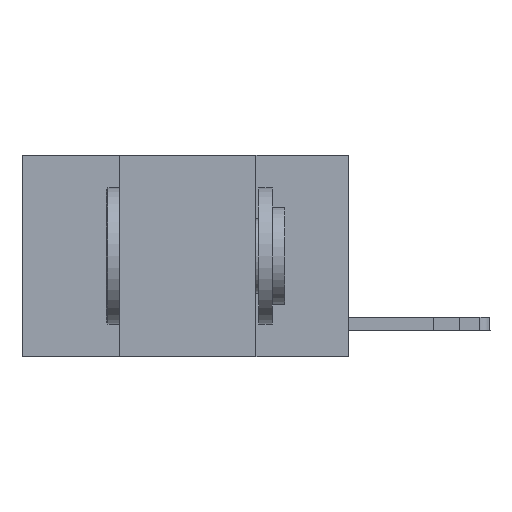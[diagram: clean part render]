
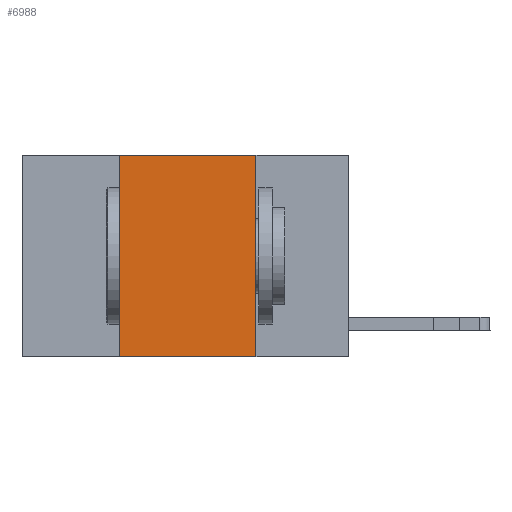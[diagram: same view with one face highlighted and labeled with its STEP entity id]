
A CAD part, left-side view. The second image highlights one B-rep face of the part: STEP entity #6988.
In plain terms, the highlighted planar face has unit normal (-1, 0, 0).
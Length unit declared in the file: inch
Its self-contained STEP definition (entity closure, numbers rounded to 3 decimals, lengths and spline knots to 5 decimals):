
#11 = CARTESIAN_POINT ( 'NONE',  ( 0., 0.17, 0. ) ) ;
#255 = DIRECTION ( 'NONE',  ( 0., 0., 1. ) ) ;
#1160 = DIRECTION ( 'NONE',  ( 0., -1., 0. ) ) ;
#1288 = DIRECTION ( 'NONE',  ( 0., 0., -1. ) ) ;
#2655 = EDGE_LOOP ( 'NONE', ( #4749, #4778, #4820, #5702 ) ) ;
#3484 = CARTESIAN_POINT ( 'NONE',  ( 0., 0.17, 0. ) ) ;
#3490 = AXIS2_PLACEMENT_3D ( 'NONE', #8842, #4213, #12386 ) ;
#3875 = LINE ( 'NONE', #14263, #12808 ) ;
#4213 = DIRECTION ( 'NONE',  ( 1., 0., 0. ) ) ;
#4749 = ORIENTED_EDGE ( 'NONE', *, *, #6648, .F. ) ;
#4778 = ORIENTED_EDGE ( 'NONE', *, *, #7293, .F. ) ;
#4820 = ORIENTED_EDGE ( 'NONE', *, *, #5601, .F. ) ;
#4833 = EDGE_CURVE ( 'NONE', #11031, #14998, #5535, .T. ) ;
#5312 = LINE ( 'NONE', #11, #13838 ) ;
#5335 = PLANE ( 'NONE',  #3490 ) ;
#5535 = LINE ( 'NONE', #6013, #11399 ) ;
#5601 = EDGE_CURVE ( 'NONE', #11031, #9595, #3875, .T. ) ;
#5702 = ORIENTED_EDGE ( 'NONE', *, *, #4833, .T. ) ;
#6013 = CARTESIAN_POINT ( 'NONE',  ( 0., 0.6, -0.37 ) ) ;
#6648 = EDGE_CURVE ( 'NONE', #11321, #14998, #5312, .T. ) ;
#6988 = ADVANCED_FACE ( 'NONE', ( #12607 ), #5335, .F. ) ;
#7153 = CARTESIAN_POINT ( 'NONE',  ( 0., 0.17, -0.37 ) ) ;
#7197 = DIRECTION ( 'NONE',  ( 0., -1., 0. ) ) ;
#7293 = EDGE_CURVE ( 'NONE', #9595, #11321, #14328, .T. ) ;
#8582 = VECTOR ( 'NONE', #1160, 39.37008 ) ;
#8842 = CARTESIAN_POINT ( 'NONE',  ( 0., 0.6, 0. ) ) ;
#9595 = VERTEX_POINT ( 'NONE', #14635 ) ;
#9938 = CARTESIAN_POINT ( 'NONE',  ( 0., 0.42, -0.37 ) ) ;
#11031 = VERTEX_POINT ( 'NONE', #9938 ) ;
#11321 = VERTEX_POINT ( 'NONE', #3484 ) ;
#11399 = VECTOR ( 'NONE', #7197, 39.37008 ) ;
#11742 = CARTESIAN_POINT ( 'NONE',  ( 0., 0.6, 0. ) ) ;
#12386 = DIRECTION ( 'NONE',  ( 0., 0., -1. ) ) ;
#12607 = FACE_OUTER_BOUND ( 'NONE', #2655, .T. ) ;
#12808 = VECTOR ( 'NONE', #255, 39.37008 ) ;
#13838 = VECTOR ( 'NONE', #1288, 39.37008 ) ;
#14263 = CARTESIAN_POINT ( 'NONE',  ( 0., 0.42, 0. ) ) ;
#14328 = LINE ( 'NONE', #11742, #8582 ) ;
#14635 = CARTESIAN_POINT ( 'NONE',  ( 0., 0.42, 0. ) ) ;
#14998 = VERTEX_POINT ( 'NONE', #7153 ) ;
